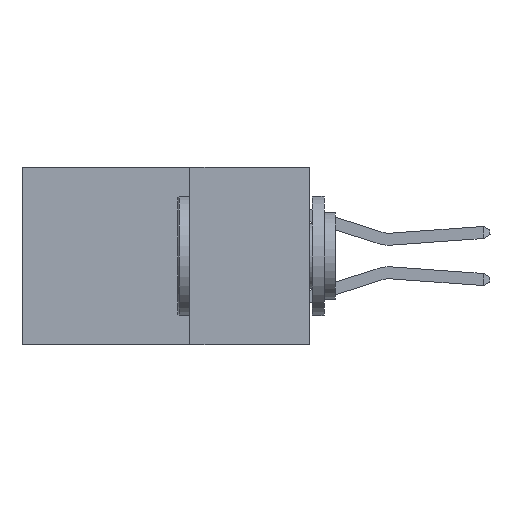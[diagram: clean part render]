
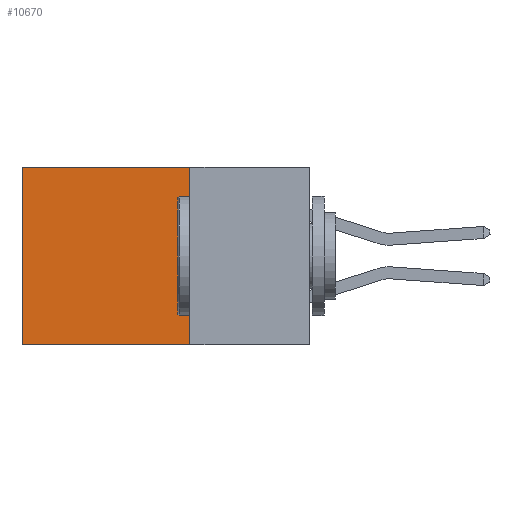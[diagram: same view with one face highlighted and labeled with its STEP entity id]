
A CAD part, left-side view. The second image highlights one B-rep face of the part: STEP entity #10670.
In plain terms, the highlighted planar face has unit normal (-1, 0, 0).
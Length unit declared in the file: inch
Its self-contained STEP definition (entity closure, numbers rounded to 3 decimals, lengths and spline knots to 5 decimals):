
#1276 = EDGE_LOOP ( 'NONE', ( #9545, #12329, #8668, #1531 ) ) ;
#1531 = ORIENTED_EDGE ( 'NONE', *, *, #6461, .T. ) ;
#1728 = VECTOR ( 'NONE', #10769, 39.37008 ) ;
#3638 = CARTESIAN_POINT ( 'NONE',  ( 0.2615, 0.6, 0. ) ) ;
#3762 = DIRECTION ( 'NONE',  ( 0., 0., -1. ) ) ;
#3788 = CARTESIAN_POINT ( 'NONE',  ( 0.2615, 0.25, -0.37 ) ) ;
#4043 = FACE_OUTER_BOUND ( 'NONE', #1276, .T. ) ;
#4072 = EDGE_CURVE ( 'NONE', #4990, #8749, #7320, .T. ) ;
#4136 = VECTOR ( 'NONE', #7010, 39.37008 ) ;
#4990 = VERTEX_POINT ( 'NONE', #3638 ) ;
#5612 = VERTEX_POINT ( 'NONE', #12353 ) ;
#6123 = AXIS2_PLACEMENT_3D ( 'NONE', #9735, #9580, #9566 ) ;
#6155 = DIRECTION ( 'NONE',  ( 0., 1., 0. ) ) ;
#6210 = CARTESIAN_POINT ( 'NONE',  ( 0.2615, 0.25, 0. ) ) ;
#6461 = EDGE_CURVE ( 'NONE', #9641, #4990, #6590, .T. ) ;
#6556 = EDGE_CURVE ( 'NONE', #9641, #5612, #8050, .T. ) ;
#6590 = LINE ( 'NONE', #6210, #9354 ) ;
#6829 = CARTESIAN_POINT ( 'NONE',  ( 0.2615, 0.6, -0.37 ) ) ;
#7010 = DIRECTION ( 'NONE',  ( 0., 0., -1. ) ) ;
#7320 = LINE ( 'NONE', #6829, #4136 ) ;
#7890 = CARTESIAN_POINT ( 'NONE',  ( 0.2615, 0.25, 0. ) ) ;
#8050 = LINE ( 'NONE', #3788, #13253 ) ;
#8668 = ORIENTED_EDGE ( 'NONE', *, *, #6556, .F. ) ;
#8749 = VERTEX_POINT ( 'NONE', #9719 ) ;
#9354 = VECTOR ( 'NONE', #6155, 39.37008 ) ;
#9545 = ORIENTED_EDGE ( 'NONE', *, *, #4072, .T. ) ;
#9556 = EDGE_CURVE ( 'NONE', #5612, #8749, #12399, .T. ) ;
#9566 = DIRECTION ( 'NONE',  ( 0., 0., -1. ) ) ;
#9580 = DIRECTION ( 'NONE',  ( 1., 0., 0. ) ) ;
#9641 = VERTEX_POINT ( 'NONE', #7890 ) ;
#9719 = CARTESIAN_POINT ( 'NONE',  ( 0.2615, 0.6, -0.37 ) ) ;
#9735 = CARTESIAN_POINT ( 'NONE',  ( 0.2615, 0.25, -0.37 ) ) ;
#9827 = PLANE ( 'NONE',  #6123 ) ;
#9845 = CARTESIAN_POINT ( 'NONE',  ( 0.2615, 0.25, -0.37 ) ) ;
#10670 = ADVANCED_FACE ( 'NONE', ( #4043 ), #9827, .F. ) ;
#10769 = DIRECTION ( 'NONE',  ( 0., 1., 0. ) ) ;
#12329 = ORIENTED_EDGE ( 'NONE', *, *, #9556, .F. ) ;
#12353 = CARTESIAN_POINT ( 'NONE',  ( 0.2615, 0.25, -0.37 ) ) ;
#12399 = LINE ( 'NONE', #9845, #1728 ) ;
#13253 = VECTOR ( 'NONE', #3762, 39.37008 ) ;
